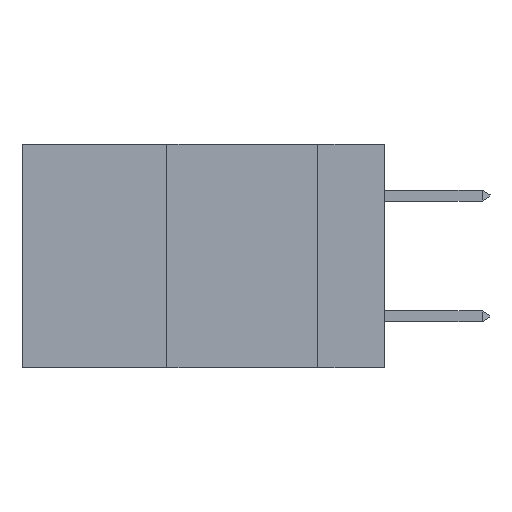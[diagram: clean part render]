
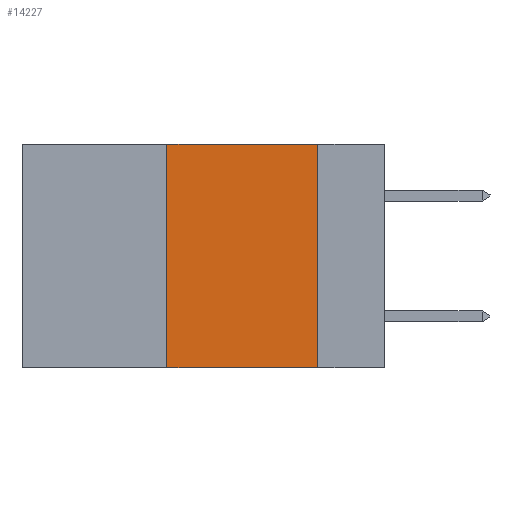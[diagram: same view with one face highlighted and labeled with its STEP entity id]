
A CAD part, left-side view. The second image highlights one B-rep face of the part: STEP entity #14227.
In plain terms, the highlighted planar face has unit normal (-1, 0, 0).
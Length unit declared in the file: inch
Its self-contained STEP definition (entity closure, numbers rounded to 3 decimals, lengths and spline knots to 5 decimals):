
#560 = EDGE_CURVE ( 'NONE', #11345, #1214, #1427, .T. ) ;
#978 = DIRECTION ( 'NONE',  ( 0., -1., 0. ) ) ;
#1063 = ORIENTED_EDGE ( 'NONE', *, *, #560, .F. ) ;
#1214 = VERTEX_POINT ( 'NONE', #5777 ) ;
#1427 = LINE ( 'NONE', #3458, #7356 ) ;
#1649 = EDGE_CURVE ( 'NONE', #11220, #3508, #2729, .T. ) ;
#2729 = LINE ( 'NONE', #10298, #8847 ) ;
#2784 = DIRECTION ( 'NONE',  ( 1., 0., 0. ) ) ;
#3182 = DIRECTION ( 'NONE',  ( 0., -1., 0. ) ) ;
#3435 = ORIENTED_EDGE ( 'NONE', *, *, #4892, .F. ) ;
#3458 = CARTESIAN_POINT ( 'NONE',  ( 0., 0.11, 0. ) ) ;
#3508 = VERTEX_POINT ( 'NONE', #12293 ) ;
#4224 = CARTESIAN_POINT ( 'NONE',  ( 0., 0.11, 0. ) ) ;
#4892 = EDGE_CURVE ( 'NONE', #3508, #11345, #10242, .T. ) ;
#5139 = AXIS2_PLACEMENT_3D ( 'NONE', #6258, #2784, #10608 ) ;
#5777 = CARTESIAN_POINT ( 'NONE',  ( 0., 0.11, -0.37 ) ) ;
#6258 = CARTESIAN_POINT ( 'NONE',  ( 0., 0.6, 0. ) ) ;
#7356 = VECTOR ( 'NONE', #11172, 39.37008 ) ;
#7428 = VECTOR ( 'NONE', #3182, 39.37008 ) ;
#7809 = FACE_OUTER_BOUND ( 'NONE', #11823, .T. ) ;
#8431 = PLANE ( 'NONE',  #5139 ) ;
#8847 = VECTOR ( 'NONE', #11925, 39.37008 ) ;
#8880 = CARTESIAN_POINT ( 'NONE',  ( 0., 0.6, 0. ) ) ;
#9518 = VECTOR ( 'NONE', #978, 39.37008 ) ;
#10242 = LINE ( 'NONE', #8880, #7428 ) ;
#10298 = CARTESIAN_POINT ( 'NONE',  ( 0., 0.36, 0. ) ) ;
#10479 = EDGE_CURVE ( 'NONE', #11220, #1214, #12527, .T. ) ;
#10608 = DIRECTION ( 'NONE',  ( 0., 0., -1. ) ) ;
#10889 = ORIENTED_EDGE ( 'NONE', *, *, #10479, .T. ) ;
#11172 = DIRECTION ( 'NONE',  ( 0., 0., -1. ) ) ;
#11220 = VERTEX_POINT ( 'NONE', #11580 ) ;
#11345 = VERTEX_POINT ( 'NONE', #4224 ) ;
#11580 = CARTESIAN_POINT ( 'NONE',  ( 0., 0.36, -0.37 ) ) ;
#11823 = EDGE_LOOP ( 'NONE', ( #1063, #3435, #13894, #10889 ) ) ;
#11925 = DIRECTION ( 'NONE',  ( 0., 0., 1. ) ) ;
#12293 = CARTESIAN_POINT ( 'NONE',  ( 0., 0.36, 0. ) ) ;
#12527 = LINE ( 'NONE', #14231, #9518 ) ;
#13894 = ORIENTED_EDGE ( 'NONE', *, *, #1649, .F. ) ;
#14227 = ADVANCED_FACE ( 'NONE', ( #7809 ), #8431, .F. ) ;
#14231 = CARTESIAN_POINT ( 'NONE',  ( 0., 0.6, -0.37 ) ) ;
